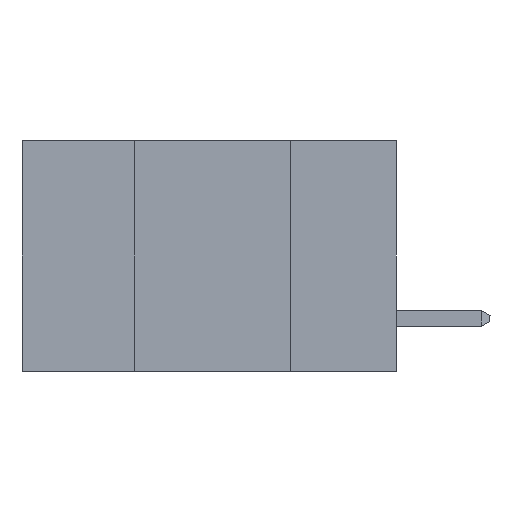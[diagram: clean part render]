
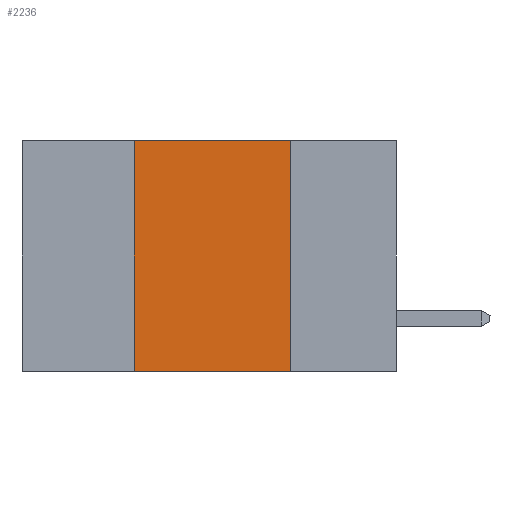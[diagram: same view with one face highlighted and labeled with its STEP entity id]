
A CAD part, left-side view. The second image highlights one B-rep face of the part: STEP entity #2236.
In plain terms, the highlighted planar face has unit normal (-1, 0, 0).
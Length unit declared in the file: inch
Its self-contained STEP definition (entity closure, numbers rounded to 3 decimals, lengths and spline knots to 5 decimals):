
#214 = CARTESIAN_POINT ( 'NONE',  ( 0., 0.17, 0. ) ) ;
#351 = CARTESIAN_POINT ( 'NONE',  ( 0., 0.42, -0.37 ) ) ;
#508 = CARTESIAN_POINT ( 'NONE',  ( 0., 0.42, -0.37 ) ) ;
#1225 = AXIS2_PLACEMENT_3D ( 'NONE', #1909, #7359, #7337 ) ;
#1263 = VECTOR ( 'NONE', #4871, 39.37008 ) ;
#1515 = EDGE_LOOP ( 'NONE', ( #2914, #6001, #4081, #4225 ) ) ;
#1909 = CARTESIAN_POINT ( 'NONE',  ( 0., 0.6, 0. ) ) ;
#1977 = VERTEX_POINT ( 'NONE', #7977 ) ;
#2236 = ADVANCED_FACE ( 'NONE', ( #2617 ), #6013, .F. ) ;
#2617 = FACE_OUTER_BOUND ( 'NONE', #1515, .T. ) ;
#2869 = VECTOR ( 'NONE', #6645, 39.37008 ) ;
#2914 = ORIENTED_EDGE ( 'NONE', *, *, #5217, .F. ) ;
#3008 = LINE ( 'NONE', #4897, #1263 ) ;
#4081 = ORIENTED_EDGE ( 'NONE', *, *, #6482, .F. ) ;
#4185 = CARTESIAN_POINT ( 'NONE',  ( 0., 0.17, -0.37 ) ) ;
#4225 = ORIENTED_EDGE ( 'NONE', *, *, #7238, .T. ) ;
#4871 = DIRECTION ( 'NONE',  ( 0., 0., -1. ) ) ;
#4897 = CARTESIAN_POINT ( 'NONE',  ( 0., 0.17, -0.37 ) ) ;
#5043 = DIRECTION ( 'NONE',  ( 0., 0., 1. ) ) ;
#5217 = EDGE_CURVE ( 'NONE', #6386, #5332, #3008, .T. ) ;
#5332 = VERTEX_POINT ( 'NONE', #4185 ) ;
#5860 = VECTOR ( 'NONE', #7844, 39.37008 ) ;
#5924 = VERTEX_POINT ( 'NONE', #508 ) ;
#6001 = ORIENTED_EDGE ( 'NONE', *, *, #6212, .F. ) ;
#6013 = PLANE ( 'NONE',  #1225 ) ;
#6046 = LINE ( 'NONE', #7176, #5860 ) ;
#6212 = EDGE_CURVE ( 'NONE', #1977, #6386, #8014, .T. ) ;
#6386 = VERTEX_POINT ( 'NONE', #214 ) ;
#6482 = EDGE_CURVE ( 'NONE', #5924, #1977, #7323, .T. ) ;
#6532 = CARTESIAN_POINT ( 'NONE',  ( 0., 0.6, 0. ) ) ;
#6645 = DIRECTION ( 'NONE',  ( 0., -1., 0. ) ) ;
#7176 = CARTESIAN_POINT ( 'NONE',  ( 0., 0.6, -0.37 ) ) ;
#7238 = EDGE_CURVE ( 'NONE', #5924, #5332, #6046, .T. ) ;
#7323 = LINE ( 'NONE', #351, #7529 ) ;
#7337 = DIRECTION ( 'NONE',  ( 0., 0., -1. ) ) ;
#7359 = DIRECTION ( 'NONE',  ( 1., 0., 0. ) ) ;
#7529 = VECTOR ( 'NONE', #5043, 39.37008 ) ;
#7844 = DIRECTION ( 'NONE',  ( 0., -1., 0. ) ) ;
#7977 = CARTESIAN_POINT ( 'NONE',  ( 0., 0.42, 0. ) ) ;
#8014 = LINE ( 'NONE', #6532, #2869 ) ;
